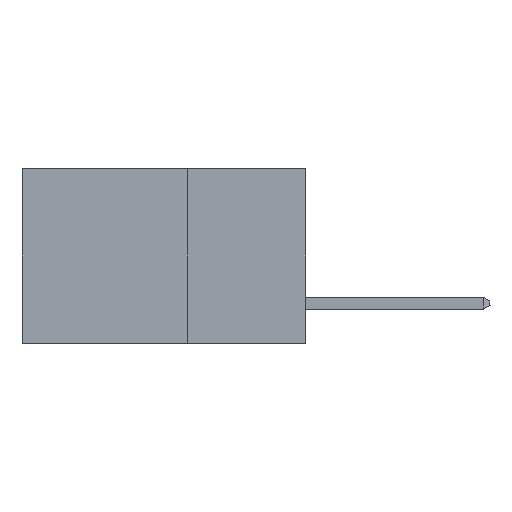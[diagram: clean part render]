
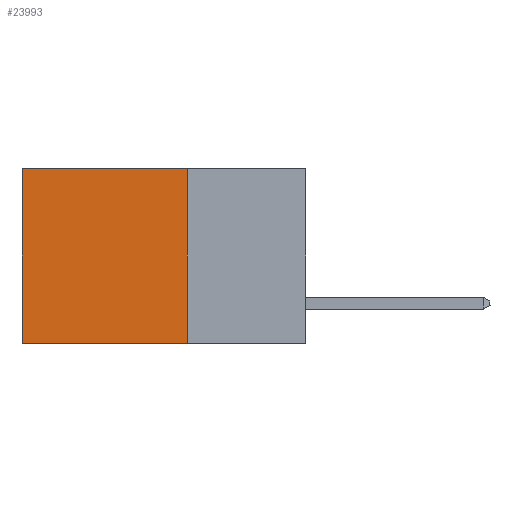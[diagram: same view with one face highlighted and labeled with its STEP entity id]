
A CAD part, left-side view. The second image highlights one B-rep face of the part: STEP entity #23993.
In plain terms, the highlighted planar face has unit normal (-1, 0, 0).
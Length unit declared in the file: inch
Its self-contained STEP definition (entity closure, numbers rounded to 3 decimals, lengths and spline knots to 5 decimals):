
#4 = DIRECTION ( 'NONE',  ( 0., 1., 0. ) ) ;
#96 = EDGE_CURVE ( 'NONE', #23532, #15945, #25265, .T. ) ;
#106 = CARTESIAN_POINT ( 'NONE',  ( 0.298, 0.25, -0.37 ) ) ;
#158 = PLANE ( 'NONE',  #16615 ) ;
#955 = CARTESIAN_POINT ( 'NONE',  ( 0.298, 0.6, 0. ) ) ;
#1784 = EDGE_LOOP ( 'NONE', ( #18070, #23346, #6434, #19625 ) ) ;
#2320 = VECTOR ( 'NONE', #5407, 39.37008 ) ;
#3712 = LINE ( 'NONE', #18517, #9770 ) ;
#3749 = VECTOR ( 'NONE', #4, 39.37008 ) ;
#5407 = DIRECTION ( 'NONE',  ( 0., 0., -1. ) ) ;
#6434 = ORIENTED_EDGE ( 'NONE', *, *, #10236, .F. ) ;
#8539 = CARTESIAN_POINT ( 'NONE',  ( 0.298, 0.25, 0. ) ) ;
#9770 = VECTOR ( 'NONE', #23572, 39.37008 ) ;
#10207 = EDGE_CURVE ( 'NONE', #15945, #19509, #10468, .T. ) ;
#10236 = EDGE_CURVE ( 'NONE', #23532, #26980, #3712, .T. ) ;
#10468 = LINE ( 'NONE', #11582, #2320 ) ;
#10509 = LINE ( 'NONE', #106, #3749 ) ;
#10980 = CARTESIAN_POINT ( 'NONE',  ( 0.298, 0.6, -0.37 ) ) ;
#11582 = CARTESIAN_POINT ( 'NONE',  ( 0.298, 0.6, 0. ) ) ;
#13743 = EDGE_CURVE ( 'NONE', #26980, #19509, #10509, .T. ) ;
#13916 = VECTOR ( 'NONE', #14806, 39.37008 ) ;
#14806 = DIRECTION ( 'NONE',  ( 0., 1., 0. ) ) ;
#15945 = VERTEX_POINT ( 'NONE', #955 ) ;
#16182 = CARTESIAN_POINT ( 'NONE',  ( 0.298, 0.25, -0.37 ) ) ;
#16615 = AXIS2_PLACEMENT_3D ( 'NONE', #20584, #20382, #17898 ) ;
#17898 = DIRECTION ( 'NONE',  ( 0., 0., -1. ) ) ;
#18070 = ORIENTED_EDGE ( 'NONE', *, *, #10207, .T. ) ;
#18517 = CARTESIAN_POINT ( 'NONE',  ( 0.298, 0.25, 0. ) ) ;
#19509 = VERTEX_POINT ( 'NONE', #10980 ) ;
#19625 = ORIENTED_EDGE ( 'NONE', *, *, #96, .T. ) ;
#20382 = DIRECTION ( 'NONE',  ( 1., 0., 0. ) ) ;
#20584 = CARTESIAN_POINT ( 'NONE',  ( 0.298, 0.25, 0. ) ) ;
#21744 = CARTESIAN_POINT ( 'NONE',  ( 0.298, 0.25, 0. ) ) ;
#23346 = ORIENTED_EDGE ( 'NONE', *, *, #13743, .F. ) ;
#23532 = VERTEX_POINT ( 'NONE', #8539 ) ;
#23572 = DIRECTION ( 'NONE',  ( 0., 0., -1. ) ) ;
#23993 = ADVANCED_FACE ( 'NONE', ( #24963 ), #158, .F. ) ;
#24963 = FACE_OUTER_BOUND ( 'NONE', #1784, .T. ) ;
#25265 = LINE ( 'NONE', #21744, #13916 ) ;
#26980 = VERTEX_POINT ( 'NONE', #16182 ) ;
